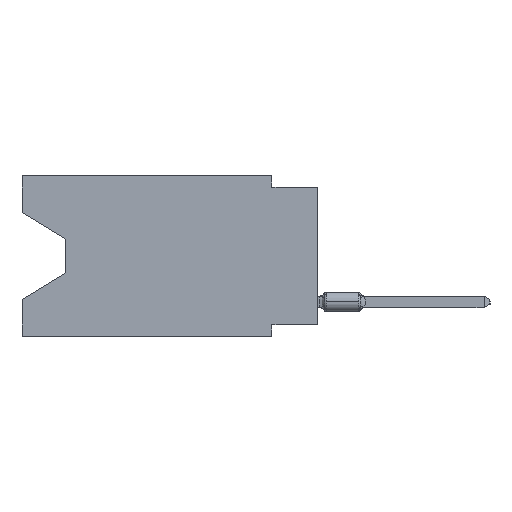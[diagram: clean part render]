
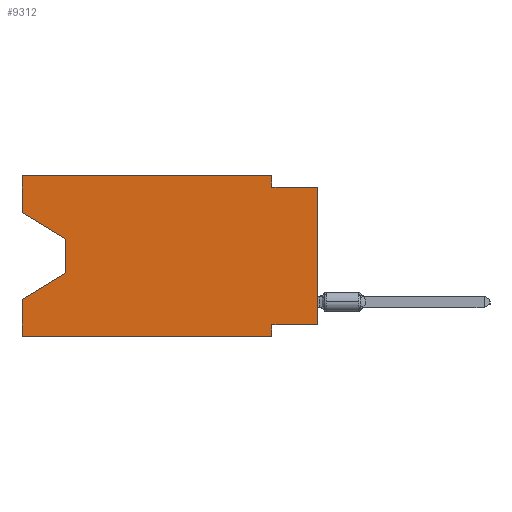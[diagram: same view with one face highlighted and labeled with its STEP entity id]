
A CAD part, left-side view. The second image highlights one B-rep face of the part: STEP entity #9312.
In plain terms, the highlighted planar face has unit normal (-1, 0, 0).
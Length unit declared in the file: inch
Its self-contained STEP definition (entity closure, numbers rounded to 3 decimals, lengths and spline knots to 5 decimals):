
#29 = CARTESIAN_POINT ( 'NONE',  ( 0., 0.1, -0.025 ) ) ;
#526 = DIRECTION ( 'NONE',  ( 0., -1., 0. ) ) ;
#1165 = VERTEX_POINT ( 'NONE', #7951 ) ;
#1290 = DIRECTION ( 'NONE',  ( 0., 0., -1. ) ) ;
#1648 = DIRECTION ( 'NONE',  ( 0., 1., 0. ) ) ;
#2420 = LINE ( 'NONE', #33777, #8055 ) ;
#3348 = DIRECTION ( 'NONE',  ( 0., -0.855, -0.519 ) ) ;
#3479 = EDGE_CURVE ( 'NONE', #1165, #6068, #26641, .T. ) ;
#4022 = ORIENTED_EDGE ( 'NONE', *, *, #23469, .T. ) ;
#4071 = VERTEX_POINT ( 'NONE', #33921 ) ;
#4656 = ORIENTED_EDGE ( 'NONE', *, *, #3479, .T. ) ;
#5140 = DIRECTION ( 'NONE',  ( 0., -1., 0. ) ) ;
#5372 = EDGE_CURVE ( 'NONE', #25107, #6553, #34715, .T. ) ;
#5864 = CARTESIAN_POINT ( 'NONE',  ( 0., 0.1, 0. ) ) ;
#6068 = VERTEX_POINT ( 'NONE', #25588 ) ;
#6248 = CARTESIAN_POINT ( 'NONE',  ( 0., 0.645, -0.08025 ) ) ;
#6324 = VECTOR ( 'NONE', #3348, 39.37008 ) ;
#6553 = VERTEX_POINT ( 'NONE', #35502 ) ;
#6592 = ORIENTED_EDGE ( 'NONE', *, *, #16165, .F. ) ;
#6812 = LINE ( 'NONE', #19551, #13710 ) ;
#7910 = LINE ( 'NONE', #20864, #10907 ) ;
#7934 = DIRECTION ( 'NONE',  ( 0., 0., -1. ) ) ;
#7951 = CARTESIAN_POINT ( 'NONE',  ( 0., 0., -0.325 ) ) ;
#8055 = VECTOR ( 'NONE', #5140, 39.37008 ) ;
#8286 = VERTEX_POINT ( 'NONE', #5864 ) ;
#9114 = AXIS2_PLACEMENT_3D ( 'NONE', #27404, #33696, #1290 ) ;
#9246 = CARTESIAN_POINT ( 'NONE',  ( 0., 0.1, -0.35 ) ) ;
#9312 = ADVANCED_FACE ( 'NONE', ( #37037 ), #20936, .F. ) ;
#10812 = VECTOR ( 'NONE', #13183, 39.37008 ) ;
#10907 = VECTOR ( 'NONE', #20660, 39.37008 ) ;
#11204 = EDGE_CURVE ( 'NONE', #1165, #14211, #26935, .T. ) ;
#11607 = CARTESIAN_POINT ( 'NONE',  ( 0., 0., 0. ) ) ;
#13183 = DIRECTION ( 'NONE',  ( 0., 0., -1. ) ) ;
#13710 = VECTOR ( 'NONE', #526, 39.37008 ) ;
#14206 = CARTESIAN_POINT ( 'NONE',  ( 0., 0.1, -0.35 ) ) ;
#14211 = VERTEX_POINT ( 'NONE', #37586 ) ;
#14297 = ORIENTED_EDGE ( 'NONE', *, *, #11204, .F. ) ;
#14669 = EDGE_CURVE ( 'NONE', #18328, #6068, #2420, .T. ) ;
#14878 = EDGE_LOOP ( 'NONE', ( #31165, #4022, #37704, #23851, #33664, #20682, #14297, #4656, #30631, #28506, #37865, #6592 ) ) ;
#15222 = DIRECTION ( 'NONE',  ( 0., 0., -1. ) ) ;
#16165 = EDGE_CURVE ( 'NONE', #25107, #36110, #7910, .T. ) ;
#16945 = CARTESIAN_POINT ( 'NONE',  ( 0., 0.55, -0.212 ) ) ;
#18206 = DIRECTION ( 'NONE',  ( 0., 0., 1. ) ) ;
#18328 = VERTEX_POINT ( 'NONE', #29 ) ;
#18481 = VECTOR ( 'NONE', #15222, 39.37008 ) ;
#18752 = CARTESIAN_POINT ( 'NONE',  ( 0., 0.1, 0. ) ) ;
#18972 = EDGE_CURVE ( 'NONE', #8286, #18328, #21480, .T. ) ;
#19551 = CARTESIAN_POINT ( 'NONE',  ( 0., 0.645, -0.35 ) ) ;
#20059 = CARTESIAN_POINT ( 'NONE',  ( 0., 0.55, -0.138 ) ) ;
#20422 = VERTEX_POINT ( 'NONE', #21680 ) ;
#20660 = DIRECTION ( 'NONE',  ( 0., 0., 1. ) ) ;
#20675 = CARTESIAN_POINT ( 'NONE',  ( 0., 0., -0.325 ) ) ;
#20682 = ORIENTED_EDGE ( 'NONE', *, *, #23649, .F. ) ;
#20864 = CARTESIAN_POINT ( 'NONE',  ( 0., 0.645, 0. ) ) ;
#20936 = PLANE ( 'NONE',  #9114 ) ;
#21480 = LINE ( 'NONE', #18752, #18481 ) ;
#21680 = CARTESIAN_POINT ( 'NONE',  ( 0., 0.645, -0.35 ) ) ;
#22992 = LINE ( 'NONE', #16945, #29399 ) ;
#23432 = VECTOR ( 'NONE', #36484, 39.37008 ) ;
#23469 = EDGE_CURVE ( 'NONE', #6553, #33109, #33016, .T. ) ;
#23649 = EDGE_CURVE ( 'NONE', #14211, #29101, #37201, .T. ) ;
#23812 = DIRECTION ( 'NONE',  ( 0., 0.855, -0.519 ) ) ;
#23851 = ORIENTED_EDGE ( 'NONE', *, *, #34667, .F. ) ;
#25107 = VERTEX_POINT ( 'NONE', #6248 ) ;
#25280 = CARTESIAN_POINT ( 'NONE',  ( 0., 0.645, 0. ) ) ;
#25588 = CARTESIAN_POINT ( 'NONE',  ( 0., 0., -0.025 ) ) ;
#26641 = LINE ( 'NONE', #11607, #23432 ) ;
#26935 = LINE ( 'NONE', #20675, #33732 ) ;
#27404 = CARTESIAN_POINT ( 'NONE',  ( 0., 0.645, 0. ) ) ;
#27498 = VECTOR ( 'NONE', #7934, 39.37008 ) ;
#27806 = CARTESIAN_POINT ( 'NONE',  ( 0., 0.645, 0. ) ) ;
#28506 = ORIENTED_EDGE ( 'NONE', *, *, #18972, .F. ) ;
#29101 = VERTEX_POINT ( 'NONE', #9246 ) ;
#29263 = EDGE_CURVE ( 'NONE', #20422, #29101, #6812, .T. ) ;
#29399 = VECTOR ( 'NONE', #23812, 39.37008 ) ;
#30631 = ORIENTED_EDGE ( 'NONE', *, *, #14669, .F. ) ;
#31165 = ORIENTED_EDGE ( 'NONE', *, *, #5372, .T. ) ;
#31171 = DIRECTION ( 'NONE',  ( 0., -1., 0. ) ) ;
#31984 = CARTESIAN_POINT ( 'NONE',  ( 0., 0.645, -0.08025 ) ) ;
#32716 = VECTOR ( 'NONE', #31171, 39.37008 ) ;
#33016 = LINE ( 'NONE', #20059, #10812 ) ;
#33109 = VERTEX_POINT ( 'NONE', #33931 ) ;
#33664 = ORIENTED_EDGE ( 'NONE', *, *, #29263, .T. ) ;
#33696 = DIRECTION ( 'NONE',  ( 1., 0., 0. ) ) ;
#33732 = VECTOR ( 'NONE', #1648, 39.37008 ) ;
#33777 = CARTESIAN_POINT ( 'NONE',  ( 0., 0., -0.025 ) ) ;
#33921 = CARTESIAN_POINT ( 'NONE',  ( 0., 0.645, -0.26975 ) ) ;
#33931 = CARTESIAN_POINT ( 'NONE',  ( 0., 0.55, -0.212 ) ) ;
#34102 = CARTESIAN_POINT ( 'NONE',  ( 0., 0.645, 0. ) ) ;
#34667 = EDGE_CURVE ( 'NONE', #20422, #4071, #39737, .T. ) ;
#34715 = LINE ( 'NONE', #31984, #6324 ) ;
#35502 = CARTESIAN_POINT ( 'NONE',  ( 0., 0.55, -0.138 ) ) ;
#35857 = EDGE_CURVE ( 'NONE', #36110, #8286, #40584, .T. ) ;
#36110 = VERTEX_POINT ( 'NONE', #25280 ) ;
#36484 = DIRECTION ( 'NONE',  ( 0., 0., 1. ) ) ;
#37037 = FACE_OUTER_BOUND ( 'NONE', #14878, .T. ) ;
#37201 = LINE ( 'NONE', #14206, #27498 ) ;
#37586 = CARTESIAN_POINT ( 'NONE',  ( 0., 0.1, -0.325 ) ) ;
#37704 = ORIENTED_EDGE ( 'NONE', *, *, #38786, .T. ) ;
#37865 = ORIENTED_EDGE ( 'NONE', *, *, #35857, .F. ) ;
#38669 = VECTOR ( 'NONE', #18206, 39.37008 ) ;
#38786 = EDGE_CURVE ( 'NONE', #33109, #4071, #22992, .T. ) ;
#39737 = LINE ( 'NONE', #27806, #38669 ) ;
#40584 = LINE ( 'NONE', #34102, #32716 ) ;
